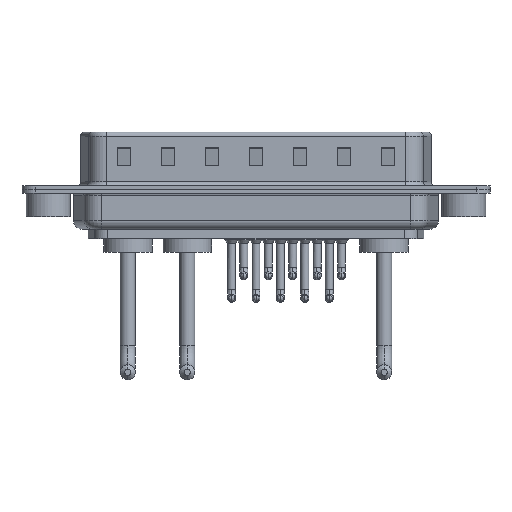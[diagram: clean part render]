
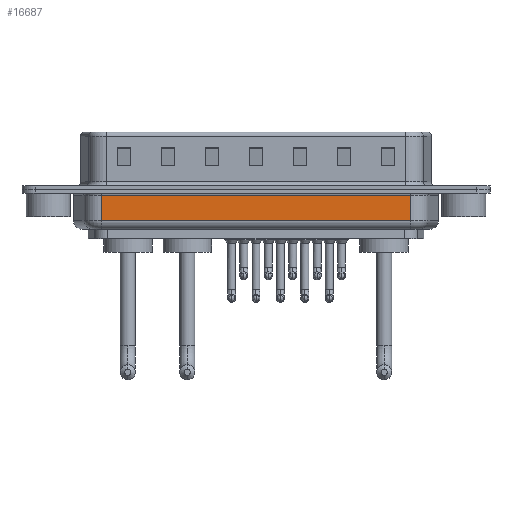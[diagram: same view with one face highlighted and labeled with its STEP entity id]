
A CAD part, front view. The second image highlights one B-rep face of the part: STEP entity #16687.
In plain terms, the highlighted planar face has unit normal (0, -1, 0).
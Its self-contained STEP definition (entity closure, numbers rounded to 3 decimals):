
#233 = LINE ( 'NONE', #14909, #3038 ) ;
#467 = VECTOR ( 'NONE', #9102, 1000. ) ;
#867 = AXIS2_PLACEMENT_3D ( 'NONE', #8603, #10645, #1541 ) ;
#1541 = DIRECTION ( 'NONE',  ( 0., 0., 1. ) ) ;
#1722 = VERTEX_POINT ( 'NONE', #14164 ) ;
#3038 = VECTOR ( 'NONE', #11357, 1000. ) ;
#3687 = VERTEX_POINT ( 'NONE', #6259 ) ;
#3830 = ORIENTED_EDGE ( 'NONE', *, *, #15263, .F. ) ;
#3928 = CARTESIAN_POINT ( 'NONE',  ( 6.006, -5.35, -0.65 ) ) ;
#5676 = DIRECTION ( 'NONE',  ( 0., 0., 1. ) ) ;
#5786 = CARTESIAN_POINT ( 'NONE',  ( 41.044, -5.35, -4.5 ) ) ;
#6259 = CARTESIAN_POINT ( 'NONE',  ( 41.044, -5.35, -0.65 ) ) ;
#6457 = CARTESIAN_POINT ( 'NONE',  ( 6.006, -5.35, -3.5 ) ) ;
#7355 = VECTOR ( 'NONE', #22574, 1000. ) ;
#7594 = LINE ( 'NONE', #5786, #15530 ) ;
#8603 = CARTESIAN_POINT ( 'NONE',  ( 6.006, -5.35, -4.5 ) ) ;
#9102 = DIRECTION ( 'NONE',  ( -1., 0., 0. ) ) ;
#9337 = LINE ( 'NONE', #3928, #467 ) ;
#9866 = VERTEX_POINT ( 'NONE', #6457 ) ;
#10645 = DIRECTION ( 'NONE',  ( 0., 1., 0. ) ) ;
#11260 = CARTESIAN_POINT ( 'NONE',  ( 41.044, -5.35, -3.5 ) ) ;
#11275 = EDGE_CURVE ( 'NONE', #9866, #19174, #233, .T. ) ;
#11357 = DIRECTION ( 'NONE',  ( 1., 0., 0. ) ) ;
#13839 = PLANE ( 'NONE',  #867 ) ;
#14164 = CARTESIAN_POINT ( 'NONE',  ( 6.006, -5.35, -0.65 ) ) ;
#14909 = CARTESIAN_POINT ( 'NONE',  ( 6.006, -5.35, -3.5 ) ) ;
#15013 = EDGE_CURVE ( 'NONE', #3687, #1722, #9337, .T. ) ;
#15263 = EDGE_CURVE ( 'NONE', #9866, #1722, #19101, .T. ) ;
#15530 = VECTOR ( 'NONE', #5676, 1000. ) ;
#16290 = ORIENTED_EDGE ( 'NONE', *, *, #15013, .T. ) ;
#16687 = ADVANCED_FACE ( 'NONE', ( #23403 ), #13839, .F. ) ;
#17292 = CARTESIAN_POINT ( 'NONE',  ( 6.006, -5.35, -4.5 ) ) ;
#19101 = LINE ( 'NONE', #17292, #7355 ) ;
#19174 = VERTEX_POINT ( 'NONE', #11260 ) ;
#21369 = EDGE_LOOP ( 'NONE', ( #3830, #22108, #22026, #16290 ) ) ;
#22026 = ORIENTED_EDGE ( 'NONE', *, *, #22855, .T. ) ;
#22108 = ORIENTED_EDGE ( 'NONE', *, *, #11275, .T. ) ;
#22574 = DIRECTION ( 'NONE',  ( 0., 0., 1. ) ) ;
#22855 = EDGE_CURVE ( 'NONE', #19174, #3687, #7594, .T. ) ;
#23403 = FACE_OUTER_BOUND ( 'NONE', #21369, .T. ) ;
